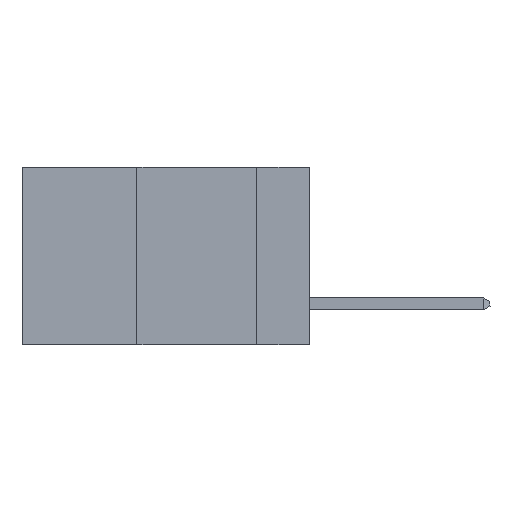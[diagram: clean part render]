
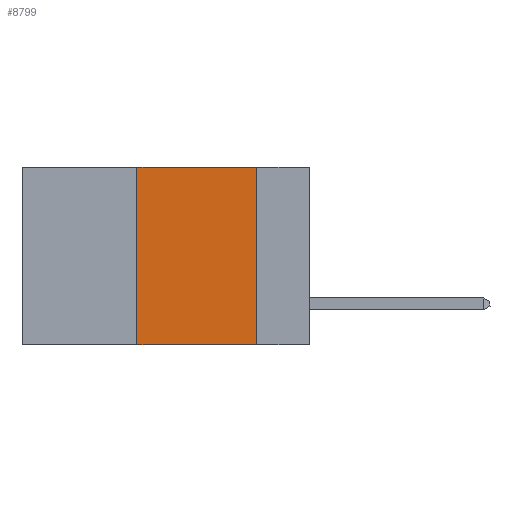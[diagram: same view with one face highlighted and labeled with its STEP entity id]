
A CAD part, left-side view. The second image highlights one B-rep face of the part: STEP entity #8799.
In plain terms, the highlighted planar face has unit normal (-1, 0, 0).
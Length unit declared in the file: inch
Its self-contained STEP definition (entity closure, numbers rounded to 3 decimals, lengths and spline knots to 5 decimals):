
#1482 = EDGE_LOOP ( 'NONE', ( #4689, #8260, #9677, #11394 ) ) ;
#1940 = CARTESIAN_POINT ( 'NONE',  ( 0., 0.6, 0. ) ) ;
#2254 = VECTOR ( 'NONE', #9776, 39.37008 ) ;
#2297 = CARTESIAN_POINT ( 'NONE',  ( 0., 0.6, 0. ) ) ;
#2623 = CARTESIAN_POINT ( 'NONE',  ( 0., 0.36, 0. ) ) ;
#3151 = VERTEX_POINT ( 'NONE', #3288 ) ;
#3288 = CARTESIAN_POINT ( 'NONE',  ( 0., 0.11, 0. ) ) ;
#3506 = EDGE_CURVE ( 'NONE', #3151, #13841, #13235, .T. ) ;
#3561 = CARTESIAN_POINT ( 'NONE',  ( 0., 0.6, -0.37 ) ) ;
#4689 = ORIENTED_EDGE ( 'NONE', *, *, #3506, .F. ) ;
#4745 = VERTEX_POINT ( 'NONE', #2623 ) ;
#4858 = CARTESIAN_POINT ( 'NONE',  ( 0., 0.36, -0.37 ) ) ;
#5137 = AXIS2_PLACEMENT_3D ( 'NONE', #2297, #11392, #9065 ) ;
#5466 = CARTESIAN_POINT ( 'NONE',  ( 0., 0.36, 0. ) ) ;
#6873 = DIRECTION ( 'NONE',  ( 0., -1., 0. ) ) ;
#7093 = LINE ( 'NONE', #5466, #7265 ) ;
#7265 = VECTOR ( 'NONE', #10231, 39.37008 ) ;
#8260 = ORIENTED_EDGE ( 'NONE', *, *, #11065, .F. ) ;
#8742 = EDGE_CURVE ( 'NONE', #10088, #13841, #11762, .T. ) ;
#8796 = VECTOR ( 'NONE', #6873, 39.37008 ) ;
#8799 = ADVANCED_FACE ( 'NONE', ( #12278 ), #12488, .F. ) ;
#9065 = DIRECTION ( 'NONE',  ( 0., 0., -1. ) ) ;
#9677 = ORIENTED_EDGE ( 'NONE', *, *, #12878, .F. ) ;
#9685 = DIRECTION ( 'NONE',  ( 0., -1., 0. ) ) ;
#9776 = DIRECTION ( 'NONE',  ( 0., 0., -1. ) ) ;
#10088 = VERTEX_POINT ( 'NONE', #4858 ) ;
#10231 = DIRECTION ( 'NONE',  ( 0., 0., 1. ) ) ;
#10898 = CARTESIAN_POINT ( 'NONE',  ( 0., 0.11, 0. ) ) ;
#11065 = EDGE_CURVE ( 'NONE', #4745, #3151, #12542, .T. ) ;
#11392 = DIRECTION ( 'NONE',  ( 1., 0., 0. ) ) ;
#11394 = ORIENTED_EDGE ( 'NONE', *, *, #8742, .T. ) ;
#11762 = LINE ( 'NONE', #3561, #8796 ) ;
#12200 = VECTOR ( 'NONE', #9685, 39.37008 ) ;
#12278 = FACE_OUTER_BOUND ( 'NONE', #1482, .T. ) ;
#12488 = PLANE ( 'NONE',  #5137 ) ;
#12542 = LINE ( 'NONE', #1940, #12200 ) ;
#12878 = EDGE_CURVE ( 'NONE', #10088, #4745, #7093, .T. ) ;
#13235 = LINE ( 'NONE', #10898, #2254 ) ;
#13841 = VERTEX_POINT ( 'NONE', #14058 ) ;
#14058 = CARTESIAN_POINT ( 'NONE',  ( 0., 0.11, -0.37 ) ) ;
